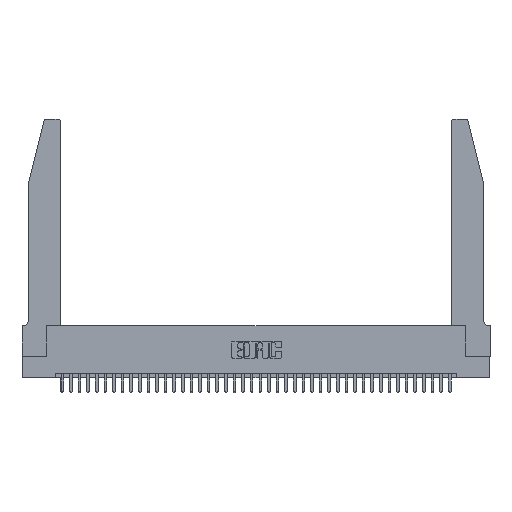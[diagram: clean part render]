
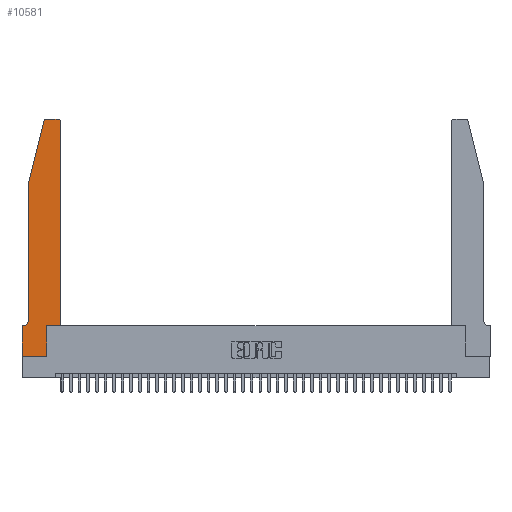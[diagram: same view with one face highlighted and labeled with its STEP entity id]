
A CAD part, top view. The second image highlights one B-rep face of the part: STEP entity #10581.
In plain terms, the highlighted planar face has unit normal (0, 0, 1).
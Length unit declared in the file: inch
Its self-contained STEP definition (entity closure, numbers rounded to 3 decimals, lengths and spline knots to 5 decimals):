
#1380 = EDGE_CURVE ( 'NONE', #37595, #37892, #20018, .T. ) ;
#1666 = CARTESIAN_POINT ( 'NONE',  ( 0., 0., 0.37 ) ) ;
#2757 = LINE ( 'NONE', #24767, #18300 ) ;
#3426 = ORIENTED_EDGE ( 'NONE', *, *, #16604, .T. ) ;
#3504 = VERTEX_POINT ( 'NONE', #16301 ) ;
#3757 = EDGE_CURVE ( 'NONE', #22138, #15474, #35498, .T. ) ;
#3978 = DIRECTION ( 'NONE',  ( 0., 0., 1. ) ) ;
#5792 = VERTEX_POINT ( 'NONE', #10559 ) ;
#5954 = EDGE_LOOP ( 'NONE', ( #3426, #36999, #10638, #22441, #12750, #24751, #35589, #8851, #24339, #32443, #6580, #15963 ) ) ;
#6136 = CIRCLE ( 'NONE', #12926, 0.07 ) ;
#6362 = DIRECTION ( 'NONE',  ( 0., 0., 1. ) ) ;
#6580 = ORIENTED_EDGE ( 'NONE', *, *, #13370, .T. ) ;
#7523 = LINE ( 'NONE', #24782, #32442 ) ;
#8851 = ORIENTED_EDGE ( 'NONE', *, *, #28808, .T. ) ;
#9297 = VECTOR ( 'NONE', #28236, 39.37008 ) ;
#9621 = CARTESIAN_POINT ( 'NONE',  ( 0.0055, 0.42, 0.37 ) ) ;
#10154 = CARTESIAN_POINT ( 'NONE',  ( 0.0755, 2., 0.37 ) ) ;
#10203 = CARTESIAN_POINT ( 'NONE',  ( 0.2865, 0.35, 0.37 ) ) ;
#10559 = CARTESIAN_POINT ( 'NONE',  ( 0.0755, 0.42, 0.37 ) ) ;
#10581 = ADVANCED_FACE ( 'NONE', ( #19551 ), #18765, .T. ) ;
#10638 = ORIENTED_EDGE ( 'NONE', *, *, #20705, .T. ) ;
#10676 = VERTEX_POINT ( 'NONE', #19025 ) ;
#10901 = CIRCLE ( 'NONE', #30538, 0.03 ) ;
#11181 = CARTESIAN_POINT ( 'NONE',  ( 0.4505, 0.35, 0.37 ) ) ;
#11331 = LINE ( 'NONE', #1666, #35344 ) ;
#12750 = ORIENTED_EDGE ( 'NONE', *, *, #37401, .T. ) ;
#12913 = CARTESIAN_POINT ( 'NONE',  ( 0.0055, 0.35, 0.37 ) ) ;
#12926 = AXIS2_PLACEMENT_3D ( 'NONE', #9621, #31511, #30806 ) ;
#12945 = CARTESIAN_POINT ( 'NONE',  ( 0., 0., 0.37 ) ) ;
#13370 = EDGE_CURVE ( 'NONE', #15474, #37595, #2757, .T. ) ;
#14254 = EDGE_CURVE ( 'NONE', #10676, #16248, #10901, .T. ) ;
#14460 = DIRECTION ( 'NONE',  ( 1., 0., 0. ) ) ;
#14617 = DIRECTION ( 'NONE',  ( 0., 0., 1. ) ) ;
#15474 = VERTEX_POINT ( 'NONE', #33302 ) ;
#15616 = CARTESIAN_POINT ( 'NONE',  ( 0.2605, 2.75, 0.37 ) ) ;
#15963 = ORIENTED_EDGE ( 'NONE', *, *, #1380, .T. ) ;
#16248 = VERTEX_POINT ( 'NONE', #21625 ) ;
#16301 = CARTESIAN_POINT ( 'NONE',  ( 0., 0.35, 0.37 ) ) ;
#16579 = CARTESIAN_POINT ( 'NONE',  ( 0.4505, 2.72, 0.37 ) ) ;
#16604 = EDGE_CURVE ( 'NONE', #37892, #10676, #25998, .T. ) ;
#16609 = LINE ( 'NONE', #21398, #23964 ) ;
#17327 = AXIS2_PLACEMENT_3D ( 'NONE', #25083, #6362, #28224 ) ;
#17978 = VERTEX_POINT ( 'NONE', #12913 ) ;
#18281 = CARTESIAN_POINT ( 'NONE',  ( 0.2865, 0., 0.37 ) ) ;
#18300 = VECTOR ( 'NONE', #27903, 39.37008 ) ;
#18765 = PLANE ( 'NONE',  #17327 ) ;
#19025 = CARTESIAN_POINT ( 'NONE',  ( 0.284, 2.75, 0.37 ) ) ;
#19422 = LINE ( 'NONE', #10154, #36019 ) ;
#19551 = FACE_OUTER_BOUND ( 'NONE', #5954, .T. ) ;
#20018 = CIRCLE ( 'NONE', #30014, 0.03 ) ;
#20253 = EDGE_CURVE ( 'NONE', #3504, #28403, #11331, .T. ) ;
#20491 = CARTESIAN_POINT ( 'NONE',  ( 0., 0., 0.37 ) ) ;
#20705 = EDGE_CURVE ( 'NONE', #16248, #33278, #35310, .T. ) ;
#21076 = CARTESIAN_POINT ( 'NONE',  ( 0.4205, 2.75, 0.37 ) ) ;
#21398 = CARTESIAN_POINT ( 'NONE',  ( 0.2865, 0.35, 0.37 ) ) ;
#21625 = CARTESIAN_POINT ( 'NONE',  ( 0.25487, 2.72718, 0.37 ) ) ;
#22138 = VERTEX_POINT ( 'NONE', #10203 ) ;
#22441 = ORIENTED_EDGE ( 'NONE', *, *, #23941, .T. ) ;
#22454 = EDGE_CURVE ( 'NONE', #30509, #22138, #16609, .T. ) ;
#22662 = CARTESIAN_POINT ( 'NONE',  ( 0.4205, 2.72, 0.37 ) ) ;
#23698 = VECTOR ( 'NONE', #25584, 39.37008 ) ;
#23941 = EDGE_CURVE ( 'NONE', #33278, #5792, #19422, .T. ) ;
#23964 = VECTOR ( 'NONE', #24555, 39.37008 ) ;
#24339 = ORIENTED_EDGE ( 'NONE', *, *, #22454, .T. ) ;
#24555 = DIRECTION ( 'NONE',  ( 0., 1., 0. ) ) ;
#24751 = ORIENTED_EDGE ( 'NONE', *, *, #38022, .T. ) ;
#24767 = CARTESIAN_POINT ( 'NONE',  ( 0.4505, 0.35, 0.37 ) ) ;
#24782 = CARTESIAN_POINT ( 'NONE',  ( 0.0755, 0.35, 0.37 ) ) ;
#25083 = CARTESIAN_POINT ( 'NONE',  ( 0., 0.35, 0.37 ) ) ;
#25531 = CARTESIAN_POINT ( 'NONE',  ( 0.0755, 2., 0.37 ) ) ;
#25584 = DIRECTION ( 'NONE',  ( 1., 0., 0. ) ) ;
#25822 = DIRECTION ( 'NONE',  ( 1., 0., 0. ) ) ;
#25998 = LINE ( 'NONE', #15616, #9297 ) ;
#27200 = VECTOR ( 'NONE', #14460, 39.37008 ) ;
#27903 = DIRECTION ( 'NONE',  ( 0., 1., 0. ) ) ;
#27923 = DIRECTION ( 'NONE',  ( -1., 0., 0. ) ) ;
#28224 = DIRECTION ( 'NONE',  ( 1., 0., 0. ) ) ;
#28236 = DIRECTION ( 'NONE',  ( -1., 0., 0. ) ) ;
#28403 = VERTEX_POINT ( 'NONE', #20491 ) ;
#28808 = EDGE_CURVE ( 'NONE', #28403, #30509, #39335, .T. ) ;
#29755 = DIRECTION ( 'NONE',  ( 0., -1., 0. ) ) ;
#30014 = AXIS2_PLACEMENT_3D ( 'NONE', #22662, #3978, #25822 ) ;
#30509 = VERTEX_POINT ( 'NONE', #18281 ) ;
#30538 = AXIS2_PLACEMENT_3D ( 'NONE', #33389, #14617, #36501 ) ;
#30806 = DIRECTION ( 'NONE',  ( -1., 0., 0. ) ) ;
#31511 = DIRECTION ( 'NONE',  ( 0., 0., -1. ) ) ;
#32442 = VECTOR ( 'NONE', #27923, 39.37008 ) ;
#32443 = ORIENTED_EDGE ( 'NONE', *, *, #3757, .T. ) ;
#33278 = VERTEX_POINT ( 'NONE', #39564 ) ;
#33302 = CARTESIAN_POINT ( 'NONE',  ( 0.4505, 0.35, 0.37 ) ) ;
#33389 = CARTESIAN_POINT ( 'NONE',  ( 0.284, 2.72, 0.37 ) ) ;
#34938 = DIRECTION ( 'NONE',  ( -0.239, -0.971, 0. ) ) ;
#35051 = DIRECTION ( 'NONE',  ( 0., -1., 0. ) ) ;
#35310 = LINE ( 'NONE', #25531, #36248 ) ;
#35344 = VECTOR ( 'NONE', #29755, 39.37008 ) ;
#35498 = LINE ( 'NONE', #11181, #27200 ) ;
#35589 = ORIENTED_EDGE ( 'NONE', *, *, #20253, .T. ) ;
#36019 = VECTOR ( 'NONE', #35051, 39.37008 ) ;
#36248 = VECTOR ( 'NONE', #34938, 39.37008 ) ;
#36501 = DIRECTION ( 'NONE',  ( 1., 0., 0. ) ) ;
#36999 = ORIENTED_EDGE ( 'NONE', *, *, #14254, .T. ) ;
#37401 = EDGE_CURVE ( 'NONE', #5792, #17978, #6136, .T. ) ;
#37595 = VERTEX_POINT ( 'NONE', #16579 ) ;
#37892 = VERTEX_POINT ( 'NONE', #21076 ) ;
#38022 = EDGE_CURVE ( 'NONE', #17978, #3504, #7523, .T. ) ;
#39335 = LINE ( 'NONE', #12945, #23698 ) ;
#39564 = CARTESIAN_POINT ( 'NONE',  ( 0.0755, 2., 0.37 ) ) ;
